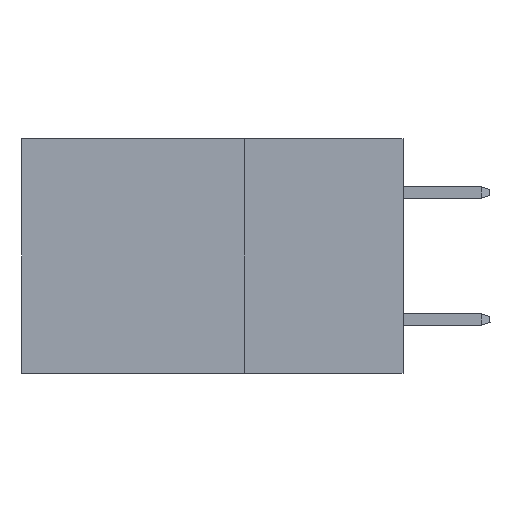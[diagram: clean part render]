
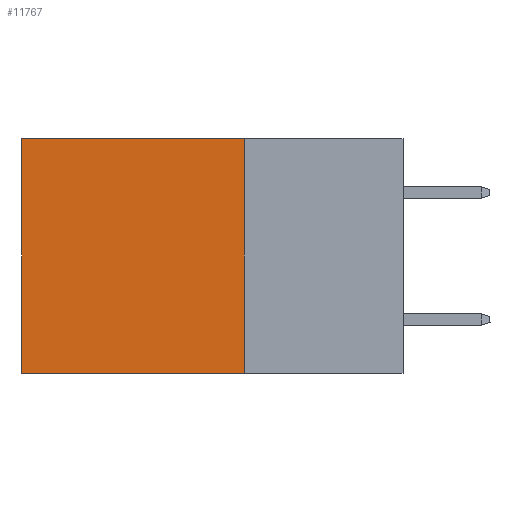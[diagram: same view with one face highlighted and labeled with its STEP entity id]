
A CAD part, left-side view. The second image highlights one B-rep face of the part: STEP entity #11767.
In plain terms, the highlighted planar face has unit normal (-1, 0, 0).
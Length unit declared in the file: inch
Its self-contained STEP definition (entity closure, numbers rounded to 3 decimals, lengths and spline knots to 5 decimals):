
#360 = DIRECTION ( 'NONE',  ( 0., 0., -1. ) ) ;
#572 = LINE ( 'NONE', #1516, #5255 ) ;
#758 = DIRECTION ( 'NONE',  ( 0., 1., 0. ) ) ;
#1049 = CARTESIAN_POINT ( 'NONE',  ( 0.2875, 0.25, -0.37 ) ) ;
#1516 = CARTESIAN_POINT ( 'NONE',  ( 0.2875, 0.25, 0. ) ) ;
#1978 = VERTEX_POINT ( 'NONE', #10507 ) ;
#2289 = EDGE_CURVE ( 'NONE', #6598, #8610, #10064, .T. ) ;
#2801 = VECTOR ( 'NONE', #360, 39.37008 ) ;
#4278 = EDGE_CURVE ( 'NONE', #6598, #1978, #572, .T. ) ;
#5255 = VECTOR ( 'NONE', #758, 39.37008 ) ;
#5586 = ORIENTED_EDGE ( 'NONE', *, *, #10328, .T. ) ;
#5701 = LINE ( 'NONE', #10318, #9150 ) ;
#5756 = ORIENTED_EDGE ( 'NONE', *, *, #4278, .T. ) ;
#5993 = ORIENTED_EDGE ( 'NONE', *, *, #8167, .F. ) ;
#6058 = FACE_OUTER_BOUND ( 'NONE', #6738, .T. ) ;
#6598 = VERTEX_POINT ( 'NONE', #11398 ) ;
#6738 = EDGE_LOOP ( 'NONE', ( #5586, #5993, #7737, #5756 ) ) ;
#7145 = CARTESIAN_POINT ( 'NONE',  ( 0.2875, 0.25, 0. ) ) ;
#7737 = ORIENTED_EDGE ( 'NONE', *, *, #2289, .F. ) ;
#8167 = EDGE_CURVE ( 'NONE', #8610, #11420, #5701, .T. ) ;
#8411 = VECTOR ( 'NONE', #11868, 39.37008 ) ;
#8610 = VERTEX_POINT ( 'NONE', #1049 ) ;
#8884 = DIRECTION ( 'NONE',  ( 1., 0., 0. ) ) ;
#9054 = CARTESIAN_POINT ( 'NONE',  ( 0.2875, 0.6, 0. ) ) ;
#9150 = VECTOR ( 'NONE', #10451, 39.37008 ) ;
#9832 = CARTESIAN_POINT ( 'NONE',  ( 0.2875, 0.25, 0. ) ) ;
#9855 = AXIS2_PLACEMENT_3D ( 'NONE', #9832, #8884, #12127 ) ;
#10011 = PLANE ( 'NONE',  #9855 ) ;
#10064 = LINE ( 'NONE', #7145, #8411 ) ;
#10318 = CARTESIAN_POINT ( 'NONE',  ( 0.2875, 0.25, -0.37 ) ) ;
#10328 = EDGE_CURVE ( 'NONE', #1978, #11420, #10829, .T. ) ;
#10451 = DIRECTION ( 'NONE',  ( 0., 1., 0. ) ) ;
#10507 = CARTESIAN_POINT ( 'NONE',  ( 0.2875, 0.6, 0. ) ) ;
#10829 = LINE ( 'NONE', #9054, #2801 ) ;
#11398 = CARTESIAN_POINT ( 'NONE',  ( 0.2875, 0.25, 0. ) ) ;
#11420 = VERTEX_POINT ( 'NONE', #11776 ) ;
#11767 = ADVANCED_FACE ( 'NONE', ( #6058 ), #10011, .F. ) ;
#11776 = CARTESIAN_POINT ( 'NONE',  ( 0.2875, 0.6, -0.37 ) ) ;
#11868 = DIRECTION ( 'NONE',  ( 0., 0., -1. ) ) ;
#12127 = DIRECTION ( 'NONE',  ( 0., 0., -1. ) ) ;
